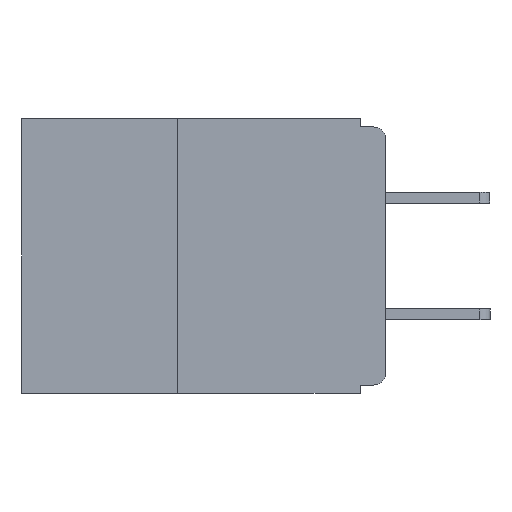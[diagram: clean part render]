
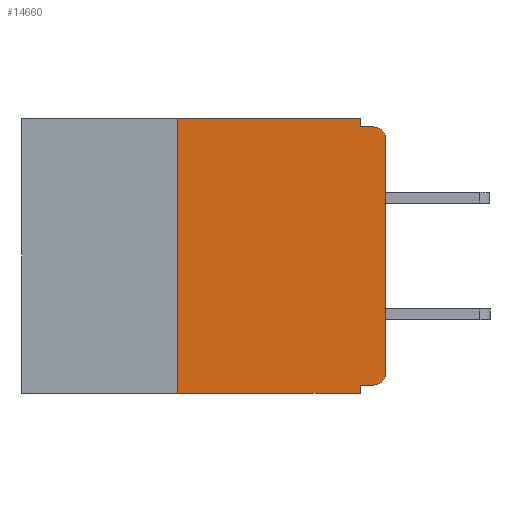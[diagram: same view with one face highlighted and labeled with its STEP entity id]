
A CAD part, left-side view. The second image highlights one B-rep face of the part: STEP entity #14660.
In plain terms, the highlighted planar face has unit normal (-1, 0, 0).
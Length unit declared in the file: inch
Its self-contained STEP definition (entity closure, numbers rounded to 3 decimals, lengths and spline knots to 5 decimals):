
#240 = DIRECTION ( 'NONE',  ( -1., 0., 0. ) ) ;
#356 = VECTOR ( 'NONE', #11215, 39.37008 ) ;
#584 = ORIENTED_EDGE ( 'NONE', *, *, #1093, .F. ) ;
#725 = VERTEX_POINT ( 'NONE', #12263 ) ;
#956 = DIRECTION ( 'NONE',  ( 1., 0., 0. ) ) ;
#1007 = VERTEX_POINT ( 'NONE', #13979 ) ;
#1035 = CARTESIAN_POINT ( 'NONE',  ( 0., 0.437, -0.33 ) ) ;
#1093 = EDGE_CURVE ( 'NONE', #12991, #7171, #8513, .T. ) ;
#1256 = CARTESIAN_POINT ( 'NONE',  ( 0., 0.031, -0.33 ) ) ;
#1435 = VERTEX_POINT ( 'NONE', #4525 ) ;
#1619 = ORIENTED_EDGE ( 'NONE', *, *, #4085, .F. ) ;
#1691 = VERTEX_POINT ( 'NONE', #4366 ) ;
#1721 = CARTESIAN_POINT ( 'NONE',  ( 0., 0., -0.01 ) ) ;
#1853 = DIRECTION ( 'NONE',  ( 0., 0., -1. ) ) ;
#2059 = VECTOR ( 'NONE', #11225, 39.37008 ) ;
#2527 = EDGE_CURVE ( 'NONE', #9083, #12152, #3709, .T. ) ;
#2767 = FACE_OUTER_BOUND ( 'NONE', #8047, .T. ) ;
#2769 = ORIENTED_EDGE ( 'NONE', *, *, #3347, .T. ) ;
#2802 = CARTESIAN_POINT ( 'NONE',  ( 0., 0.015, -0.305 ) ) ;
#2825 = CIRCLE ( 'NONE', #9378, 0.015 ) ;
#3114 = VECTOR ( 'NONE', #8090, 39.37008 ) ;
#3347 = EDGE_CURVE ( 'NONE', #1435, #9083, #4853, .T. ) ;
#3498 = CARTESIAN_POINT ( 'NONE',  ( 0., 0.031, -0.33 ) ) ;
#3709 = LINE ( 'NONE', #4953, #7511 ) ;
#3741 = LINE ( 'NONE', #8645, #356 ) ;
#3777 = VECTOR ( 'NONE', #11435, 39.37008 ) ;
#3860 = ORIENTED_EDGE ( 'NONE', *, *, #6882, .F. ) ;
#4057 = DIRECTION ( 'NONE',  ( 0., 0., -1. ) ) ;
#4085 = EDGE_CURVE ( 'NONE', #1435, #12991, #14192, .T. ) ;
#4110 = CARTESIAN_POINT ( 'NONE',  ( 0., 0.031, -0.32 ) ) ;
#4300 = CARTESIAN_POINT ( 'NONE',  ( 0., 0., -0.32 ) ) ;
#4366 = CARTESIAN_POINT ( 'NONE',  ( 0., 0.015, -0.01 ) ) ;
#4525 = CARTESIAN_POINT ( 'NONE',  ( 0., 0.015, -0.32 ) ) ;
#4684 = CARTESIAN_POINT ( 'NONE',  ( 0., 0., -0.305 ) ) ;
#4706 = VECTOR ( 'NONE', #1853, 39.37008 ) ;
#4853 = CIRCLE ( 'NONE', #8520, 0.015 ) ;
#4953 = CARTESIAN_POINT ( 'NONE',  ( 0., 0., 0. ) ) ;
#5449 = VECTOR ( 'NONE', #14388, 39.37008 ) ;
#5569 = EDGE_CURVE ( 'NONE', #12152, #1691, #2825, .T. ) ;
#5835 = LINE ( 'NONE', #1035, #2059 ) ;
#6078 = LINE ( 'NONE', #15688, #3114 ) ;
#6145 = EDGE_CURVE ( 'NONE', #1007, #9901, #7172, .T. ) ;
#6590 = CARTESIAN_POINT ( 'NONE',  ( 0., 0.25, 0. ) ) ;
#6882 = EDGE_CURVE ( 'NONE', #9901, #1691, #15584, .T. ) ;
#7171 = VERTEX_POINT ( 'NONE', #3498 ) ;
#7172 = LINE ( 'NONE', #13967, #3777 ) ;
#7334 = EDGE_CURVE ( 'NONE', #725, #7171, #5835, .T. ) ;
#7511 = VECTOR ( 'NONE', #13870, 39.37008 ) ;
#7878 = CARTESIAN_POINT ( 'NONE',  ( 0., 0.015, -0.025 ) ) ;
#8047 = EDGE_LOOP ( 'NONE', ( #10055, #12017, #3860, #8841, #8654, #13626, #8462, #584, #1619, #2769 ) ) ;
#8090 = DIRECTION ( 'NONE',  ( 0., 0., 1. ) ) ;
#8462 = ORIENTED_EDGE ( 'NONE', *, *, #7334, .T. ) ;
#8513 = LINE ( 'NONE', #1256, #4706 ) ;
#8520 = AXIS2_PLACEMENT_3D ( 'NONE', #2802, #11698, #4057 ) ;
#8645 = CARTESIAN_POINT ( 'NONE',  ( 0., 0.437, 0. ) ) ;
#8654 = ORIENTED_EDGE ( 'NONE', *, *, #10813, .F. ) ;
#8841 = ORIENTED_EDGE ( 'NONE', *, *, #6145, .F. ) ;
#9083 = VERTEX_POINT ( 'NONE', #4684 ) ;
#9171 = DIRECTION ( 'NONE',  ( 0., 0., -1. ) ) ;
#9378 = AXIS2_PLACEMENT_3D ( 'NONE', #7878, #240, #9171 ) ;
#9880 = DIRECTION ( 'NONE',  ( 0., 0., -1. ) ) ;
#9901 = VERTEX_POINT ( 'NONE', #11430 ) ;
#10055 = ORIENTED_EDGE ( 'NONE', *, *, #2527, .T. ) ;
#10448 = VECTOR ( 'NONE', #15693, 39.37008 ) ;
#10813 = EDGE_CURVE ( 'NONE', #14321, #1007, #3741, .T. ) ;
#11215 = DIRECTION ( 'NONE',  ( 0., -1., 0. ) ) ;
#11225 = DIRECTION ( 'NONE',  ( 0., -1., 0. ) ) ;
#11430 = CARTESIAN_POINT ( 'NONE',  ( 0., 0.031, -0.01 ) ) ;
#11435 = DIRECTION ( 'NONE',  ( 0., 0., -1. ) ) ;
#11698 = DIRECTION ( 'NONE',  ( -1., 0., 0. ) ) ;
#12017 = ORIENTED_EDGE ( 'NONE', *, *, #5569, .T. ) ;
#12152 = VERTEX_POINT ( 'NONE', #12580 ) ;
#12263 = CARTESIAN_POINT ( 'NONE',  ( 0., 0.25, -0.33 ) ) ;
#12350 = PLANE ( 'NONE',  #16226 ) ;
#12422 = EDGE_CURVE ( 'NONE', #725, #14321, #6078, .T. ) ;
#12580 = CARTESIAN_POINT ( 'NONE',  ( 0., 0., -0.025 ) ) ;
#12991 = VERTEX_POINT ( 'NONE', #4110 ) ;
#13626 = ORIENTED_EDGE ( 'NONE', *, *, #12422, .F. ) ;
#13870 = DIRECTION ( 'NONE',  ( 0., 0., 1. ) ) ;
#13967 = CARTESIAN_POINT ( 'NONE',  ( 0., 0.031, 0. ) ) ;
#13979 = CARTESIAN_POINT ( 'NONE',  ( 0., 0.031, 0. ) ) ;
#14192 = LINE ( 'NONE', #4300, #10448 ) ;
#14321 = VERTEX_POINT ( 'NONE', #6590 ) ;
#14388 = DIRECTION ( 'NONE',  ( 0., -1., 0. ) ) ;
#14660 = ADVANCED_FACE ( 'NONE', ( #2767 ), #12350, .F. ) ;
#14878 = CARTESIAN_POINT ( 'NONE',  ( 0., 0.437, 0. ) ) ;
#15584 = LINE ( 'NONE', #1721, #5449 ) ;
#15688 = CARTESIAN_POINT ( 'NONE',  ( 0., 0.25, -0.33 ) ) ;
#15693 = DIRECTION ( 'NONE',  ( 0., 1., 0. ) ) ;
#16226 = AXIS2_PLACEMENT_3D ( 'NONE', #14878, #956, #9880 ) ;
